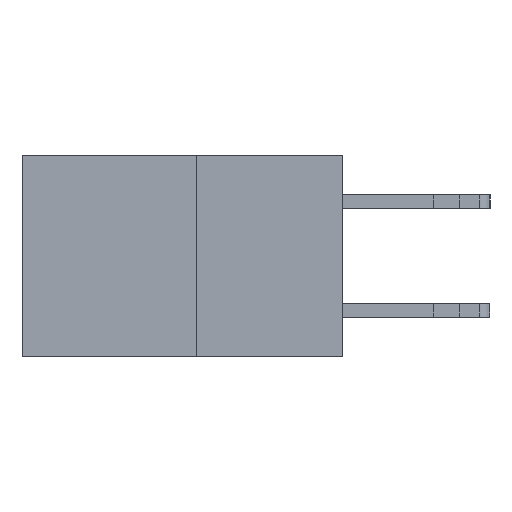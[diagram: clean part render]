
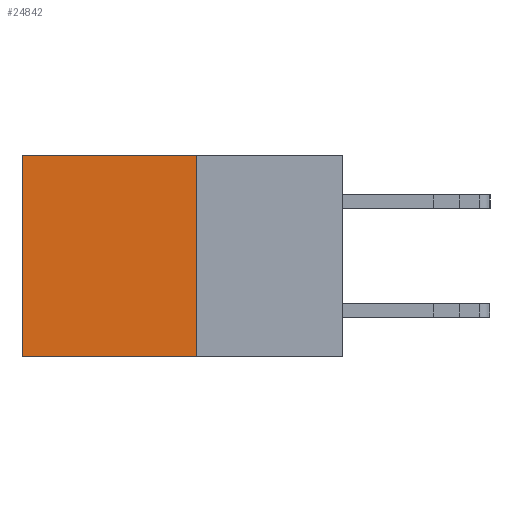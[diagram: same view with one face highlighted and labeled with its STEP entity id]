
A CAD part, left-side view. The second image highlights one B-rep face of the part: STEP entity #24842.
In plain terms, the highlighted planar face has unit normal (-1, 0, 0).
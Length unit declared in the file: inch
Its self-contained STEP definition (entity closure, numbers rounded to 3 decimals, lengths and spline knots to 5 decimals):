
#75 = VECTOR ( 'NONE', #13005, 39.37008 ) ;
#261 = EDGE_CURVE ( 'NONE', #21058, #17996, #16186, .T. ) ;
#1395 = AXIS2_PLACEMENT_3D ( 'NONE', #7226, #22710, #9538 ) ;
#1638 = CARTESIAN_POINT ( 'NONE',  ( 0.277, 0.59, 0. ) ) ;
#1904 = ORIENTED_EDGE ( 'NONE', *, *, #261, .F. ) ;
#2941 = PLANE ( 'NONE',  #1395 ) ;
#3440 = ORIENTED_EDGE ( 'NONE', *, *, #4702, .T. ) ;
#3577 = DIRECTION ( 'NONE',  ( 0., 1., 0. ) ) ;
#3718 = CARTESIAN_POINT ( 'NONE',  ( 0.277, 0.59, -0.37 ) ) ;
#4702 = EDGE_CURVE ( 'NONE', #21058, #24439, #4712, .T. ) ;
#4712 = LINE ( 'NONE', #13113, #21545 ) ;
#5468 = VECTOR ( 'NONE', #18570, 39.37008 ) ;
#5602 = CARTESIAN_POINT ( 'NONE',  ( 0.277, 0.27, -0.37 ) ) ;
#6470 = DIRECTION ( 'NONE',  ( 0., 1., 0. ) ) ;
#6772 = CARTESIAN_POINT ( 'NONE',  ( 0.277, 0.27, 0. ) ) ;
#7226 = CARTESIAN_POINT ( 'NONE',  ( 0.277, 0.27, -0.37 ) ) ;
#8591 = ORIENTED_EDGE ( 'NONE', *, *, #17904, .T. ) ;
#9538 = DIRECTION ( 'NONE',  ( 0., 0., -1. ) ) ;
#10958 = FACE_OUTER_BOUND ( 'NONE', #22106, .T. ) ;
#12541 = LINE ( 'NONE', #23248, #23529 ) ;
#13005 = DIRECTION ( 'NONE',  ( 0., 0., -1. ) ) ;
#13113 = CARTESIAN_POINT ( 'NONE',  ( 0.277, 0.27, 0. ) ) ;
#13325 = EDGE_CURVE ( 'NONE', #17996, #16364, #12541, .T. ) ;
#16186 = LINE ( 'NONE', #22413, #75 ) ;
#16353 = CARTESIAN_POINT ( 'NONE',  ( 0.277, 0.59, -0.37 ) ) ;
#16364 = VERTEX_POINT ( 'NONE', #3718 ) ;
#17904 = EDGE_CURVE ( 'NONE', #24439, #16364, #21626, .T. ) ;
#17996 = VERTEX_POINT ( 'NONE', #5602 ) ;
#18570 = DIRECTION ( 'NONE',  ( 0., 0., -1. ) ) ;
#21058 = VERTEX_POINT ( 'NONE', #6772 ) ;
#21296 = ORIENTED_EDGE ( 'NONE', *, *, #13325, .F. ) ;
#21545 = VECTOR ( 'NONE', #6470, 39.37008 ) ;
#21626 = LINE ( 'NONE', #16353, #5468 ) ;
#22106 = EDGE_LOOP ( 'NONE', ( #8591, #21296, #1904, #3440 ) ) ;
#22413 = CARTESIAN_POINT ( 'NONE',  ( 0.277, 0.27, -0.37 ) ) ;
#22710 = DIRECTION ( 'NONE',  ( 1., 0., 0. ) ) ;
#23248 = CARTESIAN_POINT ( 'NONE',  ( 0.277, 0.27, -0.37 ) ) ;
#23529 = VECTOR ( 'NONE', #3577, 39.37008 ) ;
#24439 = VERTEX_POINT ( 'NONE', #1638 ) ;
#24842 = ADVANCED_FACE ( 'NONE', ( #10958 ), #2941, .F. ) ;
